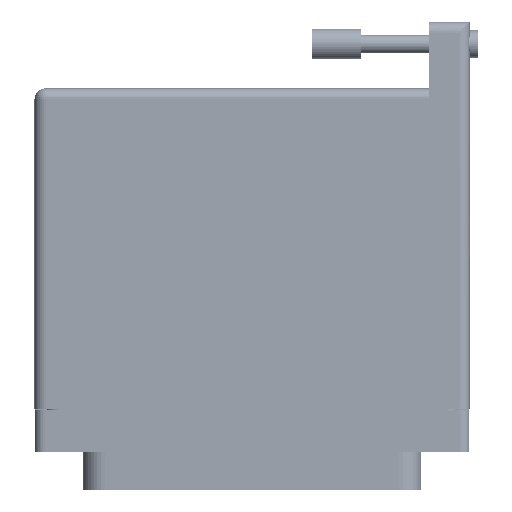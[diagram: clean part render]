
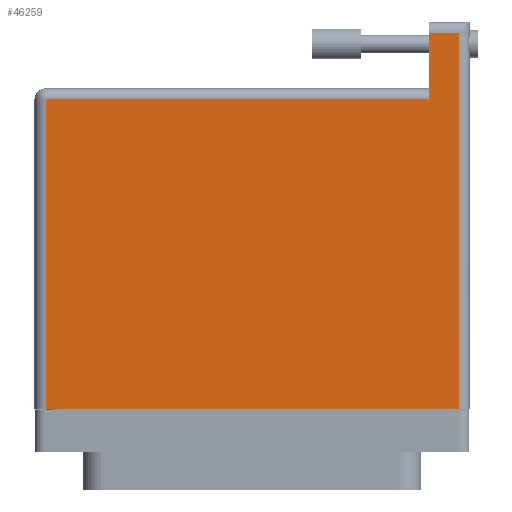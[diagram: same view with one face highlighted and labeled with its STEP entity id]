
A CAD part, front view. The second image highlights one B-rep face of the part: STEP entity #46259.
In plain terms, the highlighted face is planar.
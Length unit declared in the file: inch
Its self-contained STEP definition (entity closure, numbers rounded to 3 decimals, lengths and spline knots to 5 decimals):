
#208 = CARTESIAN_POINT ( 'NONE',  ( -1.3775, -0.1, 0.765 ) ) ;
#5158 = CARTESIAN_POINT ( 'NONE',  ( -1.3775, 1.86, 0.765 ) ) ;
#5282 = ORIENTED_EDGE ( 'NONE', *, *, #33943, .T. ) ;
#11173 = DIRECTION ( 'NONE',  ( 0., 1., 0. ) ) ;
#11621 = LINE ( 'NONE', #89686, #44040 ) ;
#14865 = LINE ( 'NONE', #208, #84284 ) ;
#17367 = DIRECTION ( 'NONE',  ( -1., 0., 0. ) ) ;
#18355 = VERTEX_POINT ( 'NONE', #26839 ) ;
#20618 = VERTEX_POINT ( 'NONE', #83249 ) ;
#26040 = AXIS2_PLACEMENT_3D ( 'NONE', #70723, #35039, #85086 ) ;
#26839 = CARTESIAN_POINT ( 'NONE',  ( 1.1215, 2.28, 0.765 ) ) ;
#27843 = DIRECTION ( 'NONE',  ( 0., -1., 0. ) ) ;
#28910 = DIRECTION ( 'NONE',  ( 1., 0., 0. ) ) ;
#29329 = CARTESIAN_POINT ( 'NONE',  ( 1.1215, 1.86, 0.765 ) ) ;
#32670 = CARTESIAN_POINT ( 'NONE',  ( -1.3075, 1.86, 0.765 ) ) ;
#32988 = VECTOR ( 'NONE', #17367, 39.37008 ) ;
#33943 = EDGE_CURVE ( 'NONE', #38060, #85254, #14865, .T. ) ;
#33954 = LINE ( 'NONE', #56672, #54225 ) ;
#34474 = DIRECTION ( 'NONE',  ( 0., -1., 0. ) ) ;
#35039 = DIRECTION ( 'NONE',  ( 0., 0., -1. ) ) ;
#35309 = LINE ( 'NONE', #91451, #68883 ) ;
#38023 = CARTESIAN_POINT ( 'NONE',  ( -1.3775, 2.28, 0.765 ) ) ;
#38060 = VERTEX_POINT ( 'NONE', #48844 ) ;
#44040 = VECTOR ( 'NONE', #11173, 39.37008 ) ;
#46259 = ADVANCED_FACE ( 'NONE', ( #50112 ), #63542, .F. ) ;
#46438 = VERTEX_POINT ( 'NONE', #32670 ) ;
#48070 = CARTESIAN_POINT ( 'NONE',  ( 1.3075, -0.1, 0.765 ) ) ;
#48269 = EDGE_CURVE ( 'NONE', #46438, #38060, #35309, .T. ) ;
#48844 = CARTESIAN_POINT ( 'NONE',  ( -1.3075, -0.1, 0.765 ) ) ;
#49803 = ORIENTED_EDGE ( 'NONE', *, *, #48269, .T. ) ;
#50112 = FACE_OUTER_BOUND ( 'NONE', #74458, .T. ) ;
#50901 = LINE ( 'NONE', #5158, #78887 ) ;
#51544 = EDGE_CURVE ( 'NONE', #56651, #46438, #50901, .T. ) ;
#54225 = VECTOR ( 'NONE', #27843, 39.37008 ) ;
#56651 = VERTEX_POINT ( 'NONE', #29329 ) ;
#56672 = CARTESIAN_POINT ( 'NONE',  ( 1.1215, 2.35, 0.765 ) ) ;
#59112 = EDGE_CURVE ( 'NONE', #20618, #18355, #73318, .T. ) ;
#59834 = ORIENTED_EDGE ( 'NONE', *, *, #86148, .T. ) ;
#63542 = PLANE ( 'NONE',  #26040 ) ;
#68883 = VECTOR ( 'NONE', #34474, 39.37008 ) ;
#70723 = CARTESIAN_POINT ( 'NONE',  ( -1.3775, 1.93, 0.765 ) ) ;
#73318 = LINE ( 'NONE', #38023, #32988 ) ;
#74458 = EDGE_LOOP ( 'NONE', ( #59834, #89956, #49803, #5282, #91341, #75762 ) ) ;
#75762 = ORIENTED_EDGE ( 'NONE', *, *, #59112, .T. ) ;
#78887 = VECTOR ( 'NONE', #89918, 39.37008 ) ;
#83249 = CARTESIAN_POINT ( 'NONE',  ( 1.3075, 2.28, 0.765 ) ) ;
#84284 = VECTOR ( 'NONE', #28910, 39.37008 ) ;
#85086 = DIRECTION ( 'NONE',  ( -1., 0., 0. ) ) ;
#85254 = VERTEX_POINT ( 'NONE', #48070 ) ;
#86148 = EDGE_CURVE ( 'NONE', #18355, #56651, #33954, .T. ) ;
#89686 = CARTESIAN_POINT ( 'NONE',  ( 1.3075, 2.35, 0.765 ) ) ;
#89918 = DIRECTION ( 'NONE',  ( -1., 0., 0. ) ) ;
#89956 = ORIENTED_EDGE ( 'NONE', *, *, #51544, .T. ) ;
#90183 = EDGE_CURVE ( 'NONE', #85254, #20618, #11621, .T. ) ;
#91341 = ORIENTED_EDGE ( 'NONE', *, *, #90183, .T. ) ;
#91451 = CARTESIAN_POINT ( 'NONE',  ( -1.3075, -0.1, 0.765 ) ) ;
